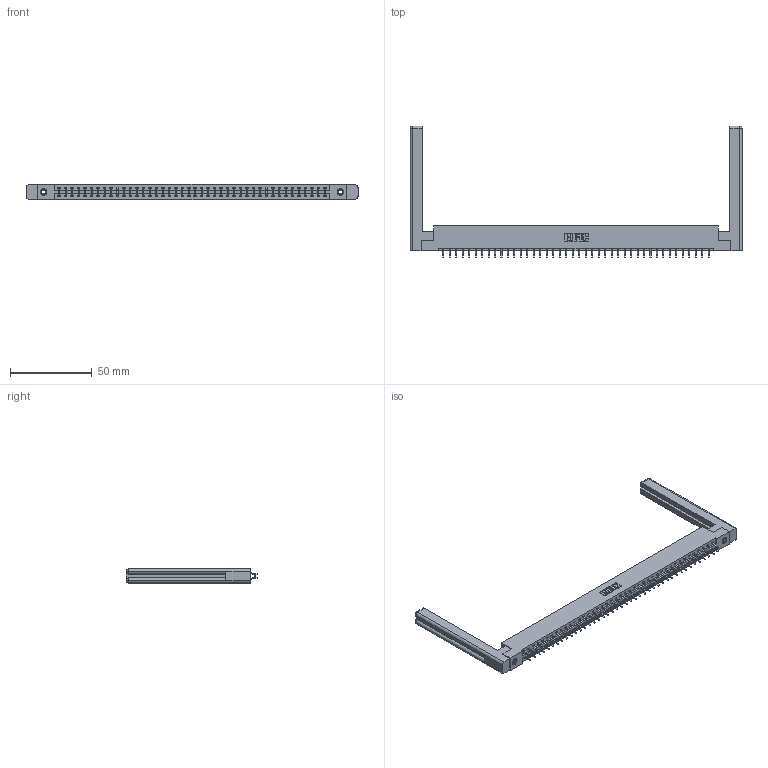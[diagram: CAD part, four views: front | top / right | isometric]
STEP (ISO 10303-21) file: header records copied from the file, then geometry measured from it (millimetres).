
FILE_DESCRIPTION (( 'STEP AP203' ), '1' );
FILE_NAME ('337-084-556-258.STEP', '2019-10-10T14:20:18', ( '' ), ( '' ), 'SwSTEP 2.0', 'SolidWorks 2016', '' );
FILE_SCHEMA (( 'CONFIG_CONTROL_DESIGN' ));
Length unit declared in the file: inch
Products named in the file (5): 307-220-058; 337 Part_Flush Mounting Lugs - 0.156 Dia-TI; 337-084-556-258; 345-250-001_345-250-001-102; 345-292-001_556 Tail
Assembly tree (89 placements, depth 2):
  337-084-556-258
    337 Part_Flush Mounting Lugs - 0.156 Dia-TI
    345-292-001_556 Tail  x84
    345-250-001_345-250-001-102  x2
    307-220-058  x2
Bounding box: 203.05 x 80.66 x 9.4 mm (x, y, z)
Volume: 28537.8 mm3; surface area: 29145.7 mm2
Topology: 89 solids, 89 shells, 5296 faces, 15701 edges, 10342 vertices
Faces by surface type: plane 3682, cylinder 1590, cone 12, torus 12
Entity records: 35418 total; most frequent: CARTESIAN_POINT 5989, ORIENTED_EDGE 5852, DIRECTION 5098, EDGE_CURVE 2926, LINE 2742, VECTOR 2742, VERTEX_POINT 1942, AXIS2_PLACEMENT_3D 1178
